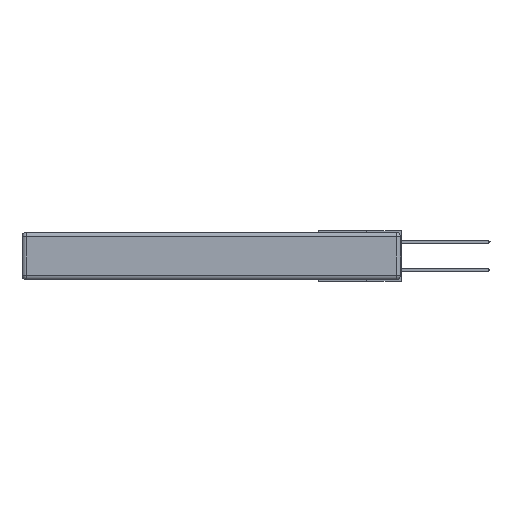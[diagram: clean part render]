
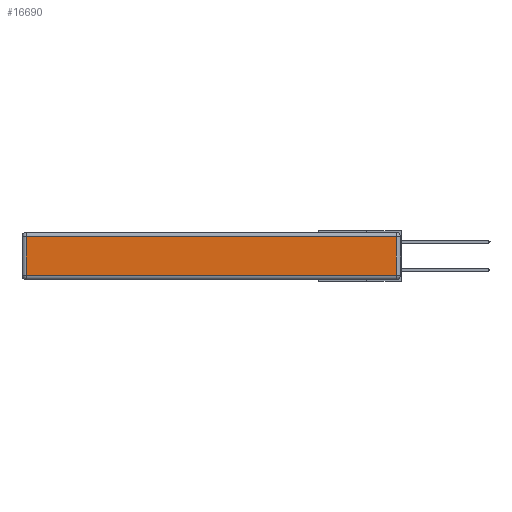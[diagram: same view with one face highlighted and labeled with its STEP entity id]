
A CAD part, left-side view. The second image highlights one B-rep face of the part: STEP entity #16690.
In plain terms, the highlighted planar face has unit normal (-1, 0, 0).
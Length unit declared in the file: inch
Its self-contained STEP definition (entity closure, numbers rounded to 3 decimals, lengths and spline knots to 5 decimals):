
#384 = CARTESIAN_POINT ( 'NONE',  ( 0., 0., -0.343 ) ) ;
#1667 = PLANE ( 'NONE',  #12501 ) ;
#2347 = ORIENTED_EDGE ( 'NONE', *, *, #3877, .T. ) ;
#2737 = CARTESIAN_POINT ( 'NONE',  ( 0., 2.72, -0.313 ) ) ;
#3025 = LINE ( 'NONE', #12864, #4470 ) ;
#3877 = EDGE_CURVE ( 'NONE', #18225, #9467, #5886, .T. ) ;
#4392 = LINE ( 'NONE', #18936, #18769 ) ;
#4470 = VECTOR ( 'NONE', #14553, 39.37008 ) ;
#5005 = DIRECTION ( 'NONE',  ( 0., -1., 0. ) ) ;
#5336 = VERTEX_POINT ( 'NONE', #5415 ) ;
#5415 = CARTESIAN_POINT ( 'NONE',  ( 0., 0.03, -0.313 ) ) ;
#5886 = LINE ( 'NONE', #10423, #9426 ) ;
#5960 = EDGE_LOOP ( 'NONE', ( #16578, #17993, #7874, #2347 ) ) ;
#6032 = FACE_OUTER_BOUND ( 'NONE', #5960, .T. ) ;
#7765 = DIRECTION ( 'NONE',  ( 0., 0., 1. ) ) ;
#7828 = EDGE_CURVE ( 'NONE', #9467, #5336, #4392, .T. ) ;
#7874 = ORIENTED_EDGE ( 'NONE', *, *, #9471, .T. ) ;
#7933 = CARTESIAN_POINT ( 'NONE',  ( 0., 0.03, -0.03 ) ) ;
#9376 = DIRECTION ( 'NONE',  ( 0., 1., 0. ) ) ;
#9426 = VECTOR ( 'NONE', #13588, 39.37008 ) ;
#9467 = VERTEX_POINT ( 'NONE', #2737 ) ;
#9471 = EDGE_CURVE ( 'NONE', #13709, #18225, #11465, .T. ) ;
#10423 = CARTESIAN_POINT ( 'NONE',  ( 0., 2.72, -0.343 ) ) ;
#10757 = VECTOR ( 'NONE', #9376, 39.37008 ) ;
#11075 = DIRECTION ( 'NONE',  ( -1., 0., 0. ) ) ;
#11465 = LINE ( 'NONE', #19740, #10757 ) ;
#12501 = AXIS2_PLACEMENT_3D ( 'NONE', #384, #11075, #7765 ) ;
#12864 = CARTESIAN_POINT ( 'NONE',  ( 0., 0.03, -0.343 ) ) ;
#13588 = DIRECTION ( 'NONE',  ( 0., 0., -1. ) ) ;
#13709 = VERTEX_POINT ( 'NONE', #7933 ) ;
#14030 = EDGE_CURVE ( 'NONE', #5336, #13709, #3025, .T. ) ;
#14553 = DIRECTION ( 'NONE',  ( 0., 0., 1. ) ) ;
#14693 = CARTESIAN_POINT ( 'NONE',  ( 0., 2.72, -0.03 ) ) ;
#16578 = ORIENTED_EDGE ( 'NONE', *, *, #7828, .T. ) ;
#16690 = ADVANCED_FACE ( 'NONE', ( #6032 ), #1667, .T. ) ;
#17993 = ORIENTED_EDGE ( 'NONE', *, *, #14030, .T. ) ;
#18225 = VERTEX_POINT ( 'NONE', #14693 ) ;
#18769 = VECTOR ( 'NONE', #5005, 39.37008 ) ;
#18936 = CARTESIAN_POINT ( 'NONE',  ( 0., 0., -0.313 ) ) ;
#19740 = CARTESIAN_POINT ( 'NONE',  ( 0., 2.75, -0.03 ) ) ;
